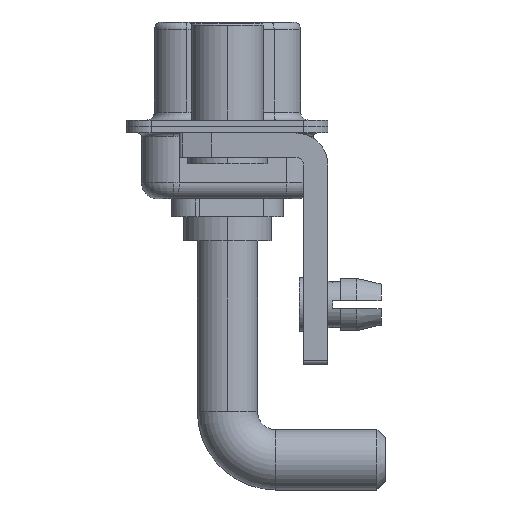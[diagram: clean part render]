
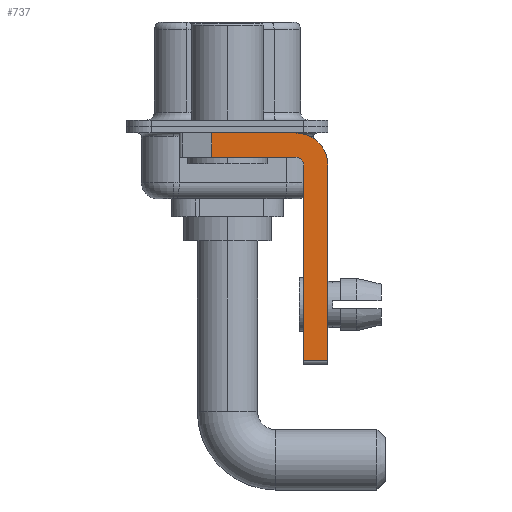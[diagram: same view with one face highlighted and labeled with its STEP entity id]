
A CAD part, left-side view. The second image highlights one B-rep face of the part: STEP entity #737.
In plain terms, the highlighted planar face has unit normal (-1, 0, 0).
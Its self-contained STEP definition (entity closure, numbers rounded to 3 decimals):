
#81 = ORIENTED_EDGE ( 'NONE', *, *, #2520, .F. ) ;
#387 = EDGE_CURVE ( 'NONE', #8866, #6290, #573, .T. ) ;
#456 = AXIS2_PLACEMENT_3D ( 'NONE', #5003, #3507, #11363 ) ;
#471 = VECTOR ( 'NONE', #12976, 1000. ) ;
#573 = LINE ( 'NONE', #669, #471 ) ;
#621 = CARTESIAN_POINT ( 'NONE',  ( -2.9, -6.25, -2.4 ) ) ;
#645 = VECTOR ( 'NONE', #11623, 1000. ) ;
#669 = CARTESIAN_POINT ( 'NONE',  ( -2.9, 0.978, -1.9 ) ) ;
#737 = ADVANCED_FACE ( 'NONE', ( #15432 ), #7678, .F. ) ;
#805 = VERTEX_POINT ( 'NONE', #12657 ) ;
#1065 = CARTESIAN_POINT ( 'NONE',  ( -2.9, -6.25, -2.4 ) ) ;
#1156 = ORIENTED_EDGE ( 'NONE', *, *, #14893, .T. ) ;
#1572 = ORIENTED_EDGE ( 'NONE', *, *, #387, .T. ) ;
#1898 = VECTOR ( 'NONE', #3084, 1000. ) ;
#2235 = EDGE_CURVE ( 'NONE', #2693, #13326, #7650, .T. ) ;
#2432 = EDGE_LOOP ( 'NONE', ( #11607, #1572, #7830, #2715, #7984, #1156, #81, #13141 ) ) ;
#2520 = EDGE_CURVE ( 'NONE', #16402, #5319, #11234, .T. ) ;
#2559 = EDGE_CURVE ( 'NONE', #7167, #16402, #15522, .T. ) ;
#2693 = VERTEX_POINT ( 'NONE', #19552 ) ;
#2715 = ORIENTED_EDGE ( 'NONE', *, *, #8332, .F. ) ;
#3084 = DIRECTION ( 'NONE',  ( 0., 0., 1. ) ) ;
#3507 = DIRECTION ( 'NONE',  ( -1., 0., 0. ) ) ;
#3644 = CARTESIAN_POINT ( 'NONE',  ( -2.9, -4.25, -1.9 ) ) ;
#3778 = DIRECTION ( 'NONE',  ( 1., 0., 0. ) ) ;
#4955 = CARTESIAN_POINT ( 'NONE',  ( -2.9, -6.25, -14.55 ) ) ;
#5003 = CARTESIAN_POINT ( 'NONE',  ( -2.9, -4.25, -2.4 ) ) ;
#5127 = CARTESIAN_POINT ( 'NONE',  ( -2.9, 0.978, -1.9 ) ) ;
#5267 = CARTESIAN_POINT ( 'NONE',  ( -2.9, -4.25, -2.4 ) ) ;
#5319 = VERTEX_POINT ( 'NONE', #4955 ) ;
#5352 = CARTESIAN_POINT ( 'NONE',  ( -2.9, -4.75, -2.4 ) ) ;
#5883 = CARTESIAN_POINT ( 'NONE',  ( -2.9, -4.25, -0.4 ) ) ;
#6101 = VECTOR ( 'NONE', #13129, 1000. ) ;
#6290 = VERTEX_POINT ( 'NONE', #5127 ) ;
#6869 = LINE ( 'NONE', #19174, #6101 ) ;
#7106 = LINE ( 'NONE', #12983, #17715 ) ;
#7167 = VERTEX_POINT ( 'NONE', #5883 ) ;
#7650 = LINE ( 'NONE', #16701, #1898 ) ;
#7678 = PLANE ( 'NONE',  #19158 ) ;
#7830 = ORIENTED_EDGE ( 'NONE', *, *, #16272, .F. ) ;
#7875 = CARTESIAN_POINT ( 'NONE',  ( -2.9, -4.25, -2.4 ) ) ;
#7984 = ORIENTED_EDGE ( 'NONE', *, *, #2235, .F. ) ;
#8049 = CIRCLE ( 'NONE', #456, 0.5 ) ;
#8332 = EDGE_CURVE ( 'NONE', #13326, #805, #8049, .T. ) ;
#8866 = VERTEX_POINT ( 'NONE', #17679 ) ;
#9264 = DIRECTION ( 'NONE',  ( 1., 0., 0. ) ) ;
#9691 = DIRECTION ( 'NONE',  ( 0., 1., 0. ) ) ;
#10183 = DIRECTION ( 'NONE',  ( 0., -1., 0. ) ) ;
#11234 = LINE ( 'NONE', #621, #645 ) ;
#11363 = DIRECTION ( 'NONE',  ( 0., 0., 1. ) ) ;
#11607 = ORIENTED_EDGE ( 'NONE', *, *, #13944, .F. ) ;
#11623 = DIRECTION ( 'NONE',  ( 0., 0., -1. ) ) ;
#12657 = CARTESIAN_POINT ( 'NONE',  ( -2.9, -4.25, -1.9 ) ) ;
#12976 = DIRECTION ( 'NONE',  ( 0., 0., -1. ) ) ;
#12983 = CARTESIAN_POINT ( 'NONE',  ( -2.9, 3., -0.4 ) ) ;
#13086 = VECTOR ( 'NONE', #9691, 1000. ) ;
#13129 = DIRECTION ( 'NONE',  ( 0., -1., 0. ) ) ;
#13141 = ORIENTED_EDGE ( 'NONE', *, *, #2559, .F. ) ;
#13326 = VERTEX_POINT ( 'NONE', #5352 ) ;
#13943 = AXIS2_PLACEMENT_3D ( 'NONE', #5267, #3778, #17475 ) ;
#13944 = EDGE_CURVE ( 'NONE', #8866, #7167, #7106, .T. ) ;
#14893 = EDGE_CURVE ( 'NONE', #2693, #5319, #6869, .T. ) ;
#15432 = FACE_OUTER_BOUND ( 'NONE', #2432, .T. ) ;
#15522 = CIRCLE ( 'NONE', #13943, 2. ) ;
#15525 = DIRECTION ( 'NONE',  ( 0., 0., -1. ) ) ;
#16272 = EDGE_CURVE ( 'NONE', #805, #6290, #17252, .T. ) ;
#16402 = VERTEX_POINT ( 'NONE', #1065 ) ;
#16701 = CARTESIAN_POINT ( 'NONE',  ( -2.9, -4.75, -14.8 ) ) ;
#17252 = LINE ( 'NONE', #3644, #13086 ) ;
#17475 = DIRECTION ( 'NONE',  ( 0., 0., -1. ) ) ;
#17679 = CARTESIAN_POINT ( 'NONE',  ( -2.9, 0.978, -0.4 ) ) ;
#17715 = VECTOR ( 'NONE', #10183, 1000. ) ;
#19158 = AXIS2_PLACEMENT_3D ( 'NONE', #7875, #9264, #15525 ) ;
#19174 = CARTESIAN_POINT ( 'NONE',  ( -2.9, -4.25, -14.55 ) ) ;
#19552 = CARTESIAN_POINT ( 'NONE',  ( -2.9, -4.75, -14.55 ) ) ;
